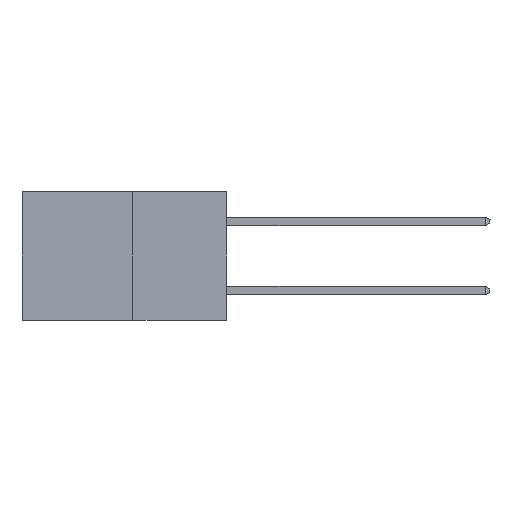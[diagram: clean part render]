
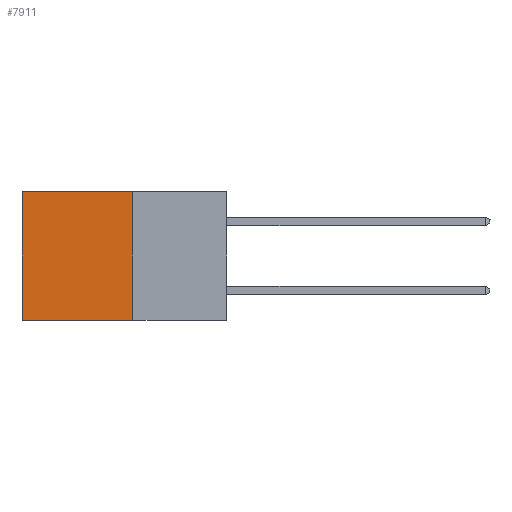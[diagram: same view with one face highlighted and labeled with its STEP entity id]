
A CAD part, left-side view. The second image highlights one B-rep face of the part: STEP entity #7911.
In plain terms, the highlighted planar face has unit normal (-1, 0, 0).
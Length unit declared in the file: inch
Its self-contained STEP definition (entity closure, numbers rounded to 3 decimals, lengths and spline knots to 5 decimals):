
#152 = VECTOR ( 'NONE', #7923, 39.37008 ) ;
#407 = EDGE_CURVE ( 'NONE', #7999, #8241, #10647, .T. ) ;
#443 = DIRECTION ( 'NONE',  ( 0., 1., 0. ) ) ;
#861 = EDGE_CURVE ( 'NONE', #3620, #7999, #10629, .T. ) ;
#1525 = VECTOR ( 'NONE', #9735, 39.37008 ) ;
#1837 = EDGE_CURVE ( 'NONE', #2206, #8241, #9368, .T. ) ;
#2167 = CARTESIAN_POINT ( 'NONE',  ( 0.277, 0.27, 0. ) ) ;
#2206 = VERTEX_POINT ( 'NONE', #10204 ) ;
#2463 = ORIENTED_EDGE ( 'NONE', *, *, #10186, .F. ) ;
#3144 = PLANE ( 'NONE',  #10637 ) ;
#3620 = VERTEX_POINT ( 'NONE', #2167 ) ;
#4143 = CARTESIAN_POINT ( 'NONE',  ( 0.277, 0.59, 0. ) ) ;
#5332 = LINE ( 'NONE', #10283, #152 ) ;
#5422 = FACE_OUTER_BOUND ( 'NONE', #7146, .T. ) ;
#5932 = CARTESIAN_POINT ( 'NONE',  ( 0.277, 0.59, -0.37 ) ) ;
#6042 = DIRECTION ( 'NONE',  ( 0., 0., -1. ) ) ;
#6449 = VECTOR ( 'NONE', #443, 39.37008 ) ;
#6776 = VECTOR ( 'NONE', #10521, 39.37008 ) ;
#6985 = ORIENTED_EDGE ( 'NONE', *, *, #407, .T. ) ;
#7146 = EDGE_LOOP ( 'NONE', ( #6985, #11107, #2463, #7243 ) ) ;
#7243 = ORIENTED_EDGE ( 'NONE', *, *, #861, .T. ) ;
#7911 = ADVANCED_FACE ( 'NONE', ( #5422 ), #3144, .F. ) ;
#7923 = DIRECTION ( 'NONE',  ( 0., 0., -1. ) ) ;
#7999 = VERTEX_POINT ( 'NONE', #4143 ) ;
#8241 = VERTEX_POINT ( 'NONE', #10245 ) ;
#8702 = CARTESIAN_POINT ( 'NONE',  ( 0.277, 0.27, 0. ) ) ;
#9236 = CARTESIAN_POINT ( 'NONE',  ( 0.277, 0.27, -0.37 ) ) ;
#9368 = LINE ( 'NONE', #11186, #6776 ) ;
#9735 = DIRECTION ( 'NONE',  ( 0., 0., -1. ) ) ;
#10186 = EDGE_CURVE ( 'NONE', #3620, #2206, #5332, .T. ) ;
#10204 = CARTESIAN_POINT ( 'NONE',  ( 0.277, 0.27, -0.37 ) ) ;
#10245 = CARTESIAN_POINT ( 'NONE',  ( 0.277, 0.59, -0.37 ) ) ;
#10283 = CARTESIAN_POINT ( 'NONE',  ( 0.277, 0.27, -0.37 ) ) ;
#10521 = DIRECTION ( 'NONE',  ( 0., 1., 0. ) ) ;
#10629 = LINE ( 'NONE', #8702, #6449 ) ;
#10637 = AXIS2_PLACEMENT_3D ( 'NONE', #9236, #10771, #6042 ) ;
#10647 = LINE ( 'NONE', #5932, #1525 ) ;
#10771 = DIRECTION ( 'NONE',  ( 1., 0., 0. ) ) ;
#11107 = ORIENTED_EDGE ( 'NONE', *, *, #1837, .F. ) ;
#11186 = CARTESIAN_POINT ( 'NONE',  ( 0.277, 0.27, -0.37 ) ) ;
